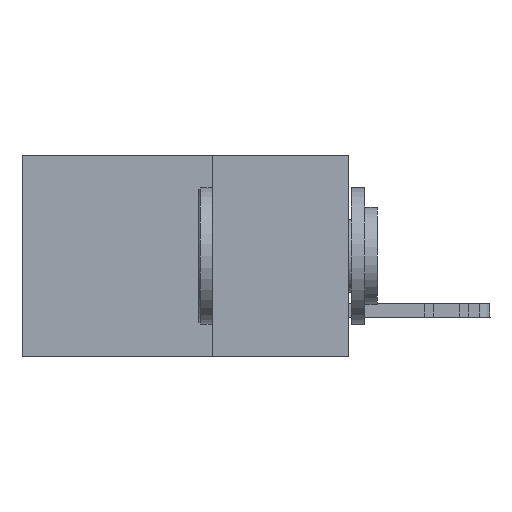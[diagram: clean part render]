
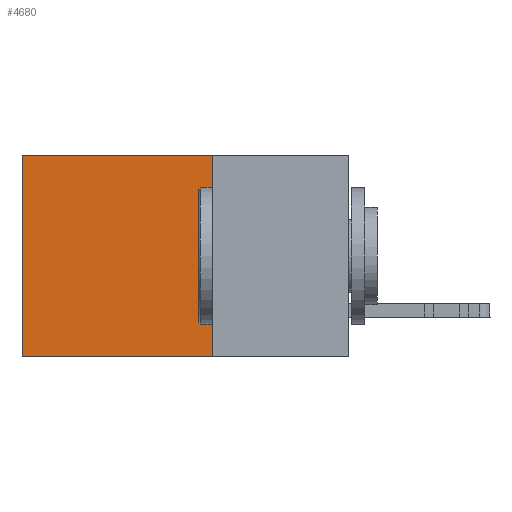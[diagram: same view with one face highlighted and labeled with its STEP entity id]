
A CAD part, left-side view. The second image highlights one B-rep face of the part: STEP entity #4680.
In plain terms, the highlighted planar face has unit normal (-1, 0, 0).
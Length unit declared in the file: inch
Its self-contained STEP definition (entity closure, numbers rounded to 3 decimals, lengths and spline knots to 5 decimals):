
#69 = VERTEX_POINT ( 'NONE', #19438 ) ;
#497 = EDGE_CURVE ( 'NONE', #69, #12177, #11840, .T. ) ;
#1944 = VERTEX_POINT ( 'NONE', #26962 ) ;
#2255 = VECTOR ( 'NONE', #15488, 39.37008 ) ;
#3631 = FACE_OUTER_BOUND ( 'NONE', #8208, .T. ) ;
#3878 = CARTESIAN_POINT ( 'NONE',  ( 0.298, 0.25, 0. ) ) ;
#4680 = ADVANCED_FACE ( 'NONE', ( #3631 ), #6237, .F. ) ;
#5510 = VECTOR ( 'NONE', #17025, 39.37008 ) ;
#6227 = VECTOR ( 'NONE', #27045, 39.37008 ) ;
#6237 = PLANE ( 'NONE',  #20131 ) ;
#6325 = DIRECTION ( 'NONE',  ( 1., 0., 0. ) ) ;
#8208 = EDGE_LOOP ( 'NONE', ( #18185, #20090, #14491, #27474 ) ) ;
#10289 = CARTESIAN_POINT ( 'NONE',  ( 0.298, 0.25, 0. ) ) ;
#11226 = CARTESIAN_POINT ( 'NONE',  ( 0.298, 0.6, 0. ) ) ;
#11840 = LINE ( 'NONE', #10289, #6227 ) ;
#12177 = VERTEX_POINT ( 'NONE', #15080 ) ;
#13512 = CARTESIAN_POINT ( 'NONE',  ( 0.298, 0.25, -0.37 ) ) ;
#14491 = ORIENTED_EDGE ( 'NONE', *, *, #19991, .F. ) ;
#15080 = CARTESIAN_POINT ( 'NONE',  ( 0.298, 0.6, 0. ) ) ;
#15488 = DIRECTION ( 'NONE',  ( 0., 0., -1. ) ) ;
#15854 = VECTOR ( 'NONE', #16283, 39.37008 ) ;
#16283 = DIRECTION ( 'NONE',  ( 0., 0., -1. ) ) ;
#16563 = CARTESIAN_POINT ( 'NONE',  ( 0.298, 0.25, 0. ) ) ;
#16931 = CARTESIAN_POINT ( 'NONE',  ( 0.298, 0.25, -0.37 ) ) ;
#17025 = DIRECTION ( 'NONE',  ( 0., 1., 0. ) ) ;
#18185 = ORIENTED_EDGE ( 'NONE', *, *, #20581, .T. ) ;
#18549 = LINE ( 'NONE', #16563, #15854 ) ;
#19438 = CARTESIAN_POINT ( 'NONE',  ( 0.298, 0.25, 0. ) ) ;
#19991 = EDGE_CURVE ( 'NONE', #69, #23083, #18549, .T. ) ;
#20090 = ORIENTED_EDGE ( 'NONE', *, *, #21455, .F. ) ;
#20131 = AXIS2_PLACEMENT_3D ( 'NONE', #3878, #6325, #27353 ) ;
#20581 = EDGE_CURVE ( 'NONE', #12177, #1944, #22817, .T. ) ;
#21072 = LINE ( 'NONE', #16931, #5510 ) ;
#21455 = EDGE_CURVE ( 'NONE', #23083, #1944, #21072, .T. ) ;
#22817 = LINE ( 'NONE', #11226, #2255 ) ;
#23083 = VERTEX_POINT ( 'NONE', #13512 ) ;
#26962 = CARTESIAN_POINT ( 'NONE',  ( 0.298, 0.6, -0.37 ) ) ;
#27045 = DIRECTION ( 'NONE',  ( 0., 1., 0. ) ) ;
#27353 = DIRECTION ( 'NONE',  ( 0., 0., -1. ) ) ;
#27474 = ORIENTED_EDGE ( 'NONE', *, *, #497, .T. ) ;
